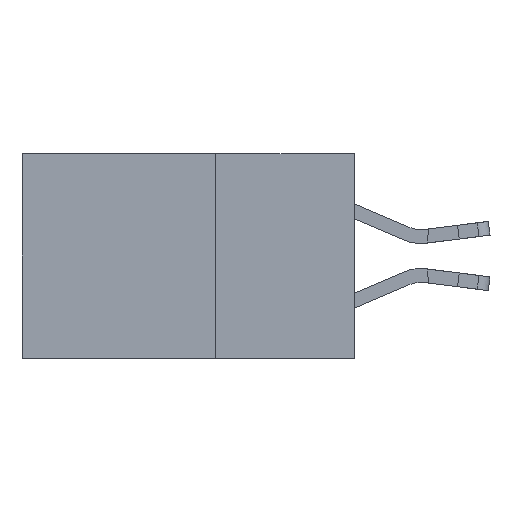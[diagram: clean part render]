
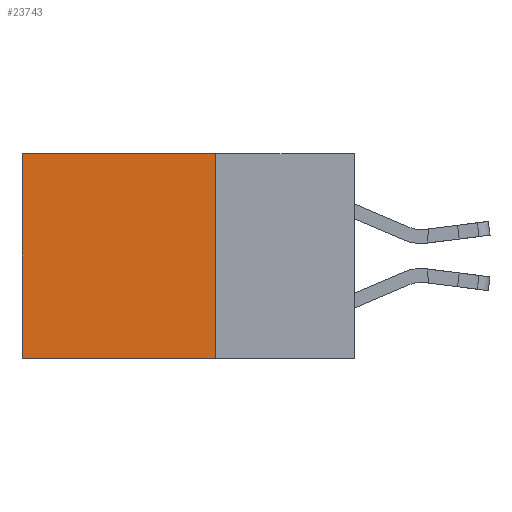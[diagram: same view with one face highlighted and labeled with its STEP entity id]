
A CAD part, left-side view. The second image highlights one B-rep face of the part: STEP entity #23743.
In plain terms, the highlighted planar face has unit normal (-1, 0, 0).
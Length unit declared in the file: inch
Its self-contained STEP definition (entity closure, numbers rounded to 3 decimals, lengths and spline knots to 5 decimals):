
#185 = CARTESIAN_POINT ( 'NONE',  ( 0.298, 0.25, -0.37 ) ) ;
#1221 = VECTOR ( 'NONE', #21142, 39.37008 ) ;
#4564 = CARTESIAN_POINT ( 'NONE',  ( 0.298, 0.25, 0. ) ) ;
#4591 = CARTESIAN_POINT ( 'NONE',  ( 0.298, 0.6, 0. ) ) ;
#7602 = EDGE_CURVE ( 'NONE', #17039, #25768, #13669, .T. ) ;
#8087 = VERTEX_POINT ( 'NONE', #4591 ) ;
#9722 = CARTESIAN_POINT ( 'NONE',  ( 0.298, 0.25, 0. ) ) ;
#10390 = ORIENTED_EDGE ( 'NONE', *, *, #12669, .T. ) ;
#10534 = VECTOR ( 'NONE', #12733, 39.37008 ) ;
#10868 = DIRECTION ( 'NONE',  ( 1., 0., 0. ) ) ;
#11144 = VECTOR ( 'NONE', #15383, 39.37008 ) ;
#12669 = EDGE_CURVE ( 'NONE', #17039, #8087, #20861, .T. ) ;
#12727 = PLANE ( 'NONE',  #14249 ) ;
#12733 = DIRECTION ( 'NONE',  ( 0., 1., 0. ) ) ;
#12813 = DIRECTION ( 'NONE',  ( 0., 0., -1. ) ) ;
#13401 = LINE ( 'NONE', #21175, #10534 ) ;
#13669 = LINE ( 'NONE', #15170, #1221 ) ;
#14249 = AXIS2_PLACEMENT_3D ( 'NONE', #4564, #10868, #12813 ) ;
#14301 = CARTESIAN_POINT ( 'NONE',  ( 0.298, 0.6, -0.37 ) ) ;
#15170 = CARTESIAN_POINT ( 'NONE',  ( 0.298, 0.25, 0. ) ) ;
#15383 = DIRECTION ( 'NONE',  ( 0., 0., -1. ) ) ;
#16179 = CARTESIAN_POINT ( 'NONE',  ( 0.298, 0.25, 0. ) ) ;
#17039 = VERTEX_POINT ( 'NONE', #16179 ) ;
#17176 = LINE ( 'NONE', #23420, #11144 ) ;
#17941 = ORIENTED_EDGE ( 'NONE', *, *, #25866, .F. ) ;
#18001 = VECTOR ( 'NONE', #26091, 39.37008 ) ;
#19266 = FACE_OUTER_BOUND ( 'NONE', #24327, .T. ) ;
#20089 = ORIENTED_EDGE ( 'NONE', *, *, #20513, .T. ) ;
#20513 = EDGE_CURVE ( 'NONE', #8087, #22400, #17176, .T. ) ;
#20861 = LINE ( 'NONE', #9722, #18001 ) ;
#20891 = ORIENTED_EDGE ( 'NONE', *, *, #7602, .F. ) ;
#21142 = DIRECTION ( 'NONE',  ( 0., 0., -1. ) ) ;
#21175 = CARTESIAN_POINT ( 'NONE',  ( 0.298, 0.25, -0.37 ) ) ;
#22400 = VERTEX_POINT ( 'NONE', #14301 ) ;
#23420 = CARTESIAN_POINT ( 'NONE',  ( 0.298, 0.6, 0. ) ) ;
#23743 = ADVANCED_FACE ( 'NONE', ( #19266 ), #12727, .F. ) ;
#24327 = EDGE_LOOP ( 'NONE', ( #20089, #17941, #20891, #10390 ) ) ;
#25768 = VERTEX_POINT ( 'NONE', #185 ) ;
#25866 = EDGE_CURVE ( 'NONE', #25768, #22400, #13401, .T. ) ;
#26091 = DIRECTION ( 'NONE',  ( 0., 1., 0. ) ) ;
